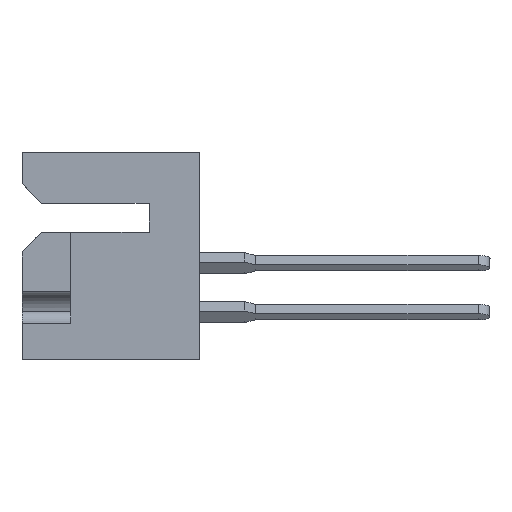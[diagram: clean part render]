
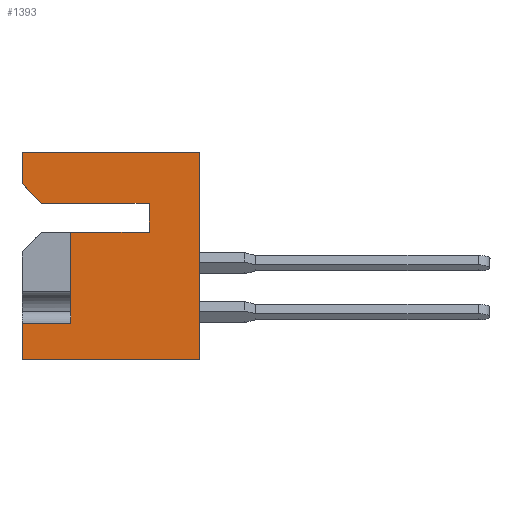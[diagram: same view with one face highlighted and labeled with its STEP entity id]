
A CAD part, left-side view. The second image highlights one B-rep face of the part: STEP entity #1393.
In plain terms, the highlighted planar face has unit normal (-1, 0, 0).
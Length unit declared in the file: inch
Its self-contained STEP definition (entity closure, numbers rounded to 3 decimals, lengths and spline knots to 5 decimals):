
#208 = CARTESIAN_POINT ( 'NONE',  ( 0., 0.128, -0.205 ) ) ;
#410 = ORIENTED_EDGE ( 'NONE', *, *, #10064, .F. ) ;
#517 = EDGE_CURVE ( 'NONE', #10603, #20306, #8395, .T. ) ;
#1269 = CARTESIAN_POINT ( 'NONE',  ( 0., 0.453, 0. ) ) ;
#1393 = ADVANCED_FACE ( 'NONE', ( #16564 ), #15947, .F. ) ;
#1705 = CARTESIAN_POINT ( 'NONE',  ( 0., 0.453, 0. ) ) ;
#1800 = CARTESIAN_POINT ( 'NONE',  ( 0., 0.328, -0.205 ) ) ;
#1841 = VERTEX_POINT ( 'NONE', #1269 ) ;
#2228 = EDGE_LOOP ( 'NONE', ( #30785, #28634, #10770, #25213, #27651, #410, #12169, #30020, #6777, #30484, #7739 ) ) ;
#2396 = CARTESIAN_POINT ( 'NONE',  ( 0., 0.128, -0.131 ) ) ;
#4532 = VERTEX_POINT ( 'NONE', #23104 ) ;
#4664 = LINE ( 'NONE', #10487, #17329 ) ;
#4991 = DIRECTION ( 'NONE',  ( 0., -1., 0. ) ) ;
#6031 = CARTESIAN_POINT ( 'NONE',  ( 0., 0.453, -0.531 ) ) ;
#6151 = CARTESIAN_POINT ( 'NONE',  ( 0., 0.403, -0.131 ) ) ;
#6224 = DIRECTION ( 'NONE',  ( 0., -1., 0. ) ) ;
#6342 = DIRECTION ( 'NONE',  ( 0., -0.707, -0.707 ) ) ;
#6499 = EDGE_CURVE ( 'NONE', #4532, #29660, #9401, .T. ) ;
#6659 = CARTESIAN_POINT ( 'NONE',  ( 0., 0.128, -0.131 ) ) ;
#6777 = ORIENTED_EDGE ( 'NONE', *, *, #12337, .F. ) ;
#7304 = CARTESIAN_POINT ( 'NONE',  ( 0., 0.128, -0.131 ) ) ;
#7739 = ORIENTED_EDGE ( 'NONE', *, *, #13402, .F. ) ;
#7872 = CARTESIAN_POINT ( 'NONE',  ( 0., 0.453, 0. ) ) ;
#8022 = VERTEX_POINT ( 'NONE', #16206 ) ;
#8199 = CARTESIAN_POINT ( 'NONE',  ( 0., 0., 0. ) ) ;
#8369 = LINE ( 'NONE', #208, #28407 ) ;
#8395 = LINE ( 'NONE', #2396, #12113 ) ;
#8963 = CARTESIAN_POINT ( 'NONE',  ( 0., 0., -0.531 ) ) ;
#9033 = VECTOR ( 'NONE', #6224, 39.37008 ) ;
#9401 = LINE ( 'NONE', #13393, #24261 ) ;
#9469 = DIRECTION ( 'NONE',  ( 0., 0., 1. ) ) ;
#9477 = CARTESIAN_POINT ( 'NONE',  ( 0., 0.453, 0. ) ) ;
#10064 = EDGE_CURVE ( 'NONE', #8022, #1841, #4664, .T. ) ;
#10487 = CARTESIAN_POINT ( 'NONE',  ( 0., 0.453, 0. ) ) ;
#10603 = VERTEX_POINT ( 'NONE', #7304 ) ;
#10770 = ORIENTED_EDGE ( 'NONE', *, *, #17063, .T. ) ;
#10993 = DIRECTION ( 'NONE',  ( 1., 0., 0. ) ) ;
#11470 = CARTESIAN_POINT ( 'NONE',  ( 0., 0.128, -0.205 ) ) ;
#11870 = CARTESIAN_POINT ( 'NONE',  ( 0., 0.403, -0.131 ) ) ;
#12113 = VECTOR ( 'NONE', #23580, 39.37008 ) ;
#12150 = VECTOR ( 'NONE', #4991, 39.37008 ) ;
#12169 = ORIENTED_EDGE ( 'NONE', *, *, #12210, .T. ) ;
#12210 = EDGE_CURVE ( 'NONE', #8022, #20306, #12557, .T. ) ;
#12337 = EDGE_CURVE ( 'NONE', #19442, #10603, #29675, .T. ) ;
#12520 = VECTOR ( 'NONE', #9469, 39.37008 ) ;
#12557 = LINE ( 'NONE', #6151, #16651 ) ;
#12998 = CARTESIAN_POINT ( 'NONE',  ( 0., 0.453, -0.437 ) ) ;
#13231 = LINE ( 'NONE', #1800, #19567 ) ;
#13393 = CARTESIAN_POINT ( 'NONE',  ( 0., 0.328, -0.437 ) ) ;
#13402 = EDGE_CURVE ( 'NONE', #4532, #21149, #13231, .T. ) ;
#14681 = DIRECTION ( 'NONE',  ( 0., 0., 1. ) ) ;
#14896 = LINE ( 'NONE', #7872, #15648 ) ;
#15648 = VECTOR ( 'NONE', #14681, 39.37008 ) ;
#15671 = CARTESIAN_POINT ( 'NONE',  ( 0., 0.453, -0.531 ) ) ;
#15947 = PLANE ( 'NONE',  #25229 ) ;
#16206 = CARTESIAN_POINT ( 'NONE',  ( 0., 0.453, -0.081 ) ) ;
#16464 = VECTOR ( 'NONE', #18450, 39.37008 ) ;
#16564 = FACE_OUTER_BOUND ( 'NONE', #2228, .T. ) ;
#16651 = VECTOR ( 'NONE', #6342, 39.37008 ) ;
#17063 = EDGE_CURVE ( 'NONE', #18735, #19350, #22769, .T. ) ;
#17329 = VECTOR ( 'NONE', #29402, 39.37008 ) ;
#18450 = DIRECTION ( 'NONE',  ( 0., 0., 1. ) ) ;
#18735 = VERTEX_POINT ( 'NONE', #6031 ) ;
#19350 = VERTEX_POINT ( 'NONE', #8963 ) ;
#19442 = VERTEX_POINT ( 'NONE', #11470 ) ;
#19567 = VECTOR ( 'NONE', #30085, 39.37008 ) ;
#19805 = LINE ( 'NONE', #27865, #16464 ) ;
#20306 = VERTEX_POINT ( 'NONE', #11870 ) ;
#20354 = EDGE_CURVE ( 'NONE', #1841, #28129, #24785, .T. ) ;
#21149 = VERTEX_POINT ( 'NONE', #29473 ) ;
#21638 = DIRECTION ( 'NONE',  ( 0., 1., 0. ) ) ;
#22651 = DIRECTION ( 'NONE',  ( 0., 1., 0. ) ) ;
#22769 = LINE ( 'NONE', #15671, #9033 ) ;
#23104 = CARTESIAN_POINT ( 'NONE',  ( 0., 0.328, -0.437 ) ) ;
#23580 = DIRECTION ( 'NONE',  ( 0., 1., 0. ) ) ;
#23812 = EDGE_CURVE ( 'NONE', #19442, #21149, #8369, .T. ) ;
#24261 = VECTOR ( 'NONE', #22651, 39.37008 ) ;
#24785 = LINE ( 'NONE', #9477, #12150 ) ;
#25213 = ORIENTED_EDGE ( 'NONE', *, *, #29839, .T. ) ;
#25229 = AXIS2_PLACEMENT_3D ( 'NONE', #1705, #10993, #27587 ) ;
#25935 = EDGE_CURVE ( 'NONE', #18735, #29660, #14896, .T. ) ;
#27587 = DIRECTION ( 'NONE',  ( 0., 0., -1. ) ) ;
#27651 = ORIENTED_EDGE ( 'NONE', *, *, #20354, .F. ) ;
#27865 = CARTESIAN_POINT ( 'NONE',  ( 0., 0., 0. ) ) ;
#28129 = VERTEX_POINT ( 'NONE', #8199 ) ;
#28407 = VECTOR ( 'NONE', #21638, 39.37008 ) ;
#28634 = ORIENTED_EDGE ( 'NONE', *, *, #25935, .F. ) ;
#29402 = DIRECTION ( 'NONE',  ( 0., 0., 1. ) ) ;
#29473 = CARTESIAN_POINT ( 'NONE',  ( 0., 0.328, -0.205 ) ) ;
#29660 = VERTEX_POINT ( 'NONE', #12998 ) ;
#29675 = LINE ( 'NONE', #6659, #12520 ) ;
#29839 = EDGE_CURVE ( 'NONE', #19350, #28129, #19805, .T. ) ;
#30020 = ORIENTED_EDGE ( 'NONE', *, *, #517, .F. ) ;
#30085 = DIRECTION ( 'NONE',  ( 0., 0., 1. ) ) ;
#30484 = ORIENTED_EDGE ( 'NONE', *, *, #23812, .T. ) ;
#30785 = ORIENTED_EDGE ( 'NONE', *, *, #6499, .T. ) ;
